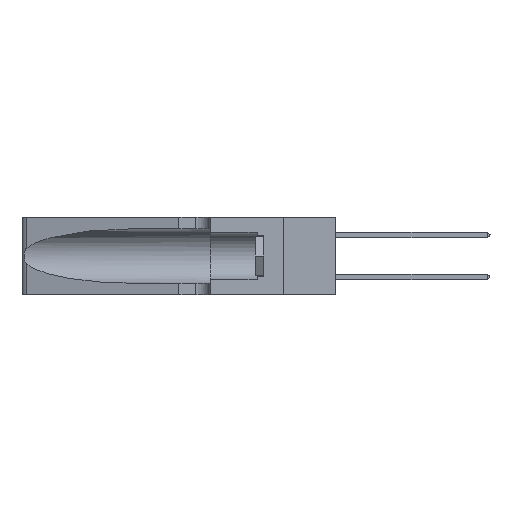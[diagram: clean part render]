
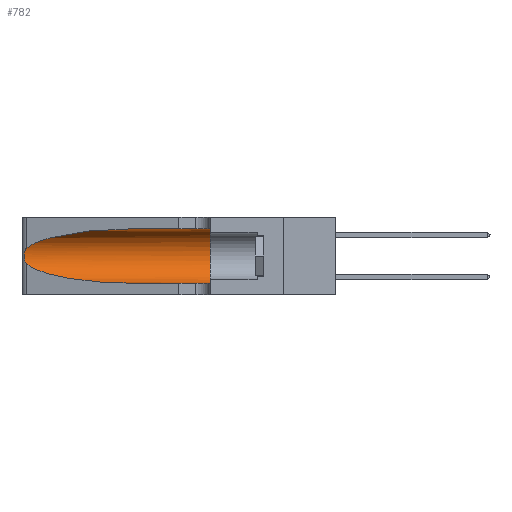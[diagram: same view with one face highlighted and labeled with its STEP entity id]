
A CAD part, left-side view. The second image highlights one B-rep face of the part: STEP entity #782.
In plain terms, the highlighted cylindrical face has radius 3.308 mm (diameter 6.617 mm), a partial arc.
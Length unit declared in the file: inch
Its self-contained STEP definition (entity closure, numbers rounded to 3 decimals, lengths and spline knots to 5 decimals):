
#251 =( BOUNDED_CURVE ( )  B_SPLINE_CURVE ( 3, ( #7441, #18581, #9329, #22350 ),
 .UNSPECIFIED., .F., .F. ) 
 B_SPLINE_CURVE_WITH_KNOTS ( ( 4, 4 ),
 ( 3.44316, 4.71239 ),
 .UNSPECIFIED. ) 
 CURVE ( )  GEOMETRIC_REPRESENTATION_ITEM ( )  RATIONAL_B_SPLINE_CURVE ( ( 1., 0.87, 0.87, 1. ) ) 
 REPRESENTATION_ITEM ( '' )  );
#782 = ADVANCED_FACE ( 'NONE', ( #13911 ), #3469, .F. ) ;
#1122 = VERTEX_POINT ( 'NONE', #4785 ) ;
#1223 = LINE ( 'NONE', #7071, #16036 ) ;
#1306 = ORIENTED_EDGE ( 'NONE', *, *, #3313, .T. ) ;
#1333 = CARTESIAN_POINT ( 'NONE',  ( 0.26075, 1.23896, 0.178 ) ) ;
#2041 =( BOUNDED_CURVE ( )  B_SPLINE_CURVE ( 3, ( #22969, #21087, #9941, #11788 ),
 .UNSPECIFIED., .F., .T. ) 
 B_SPLINE_CURVE_WITH_KNOTS ( ( 4, 4 ),
 ( 1.5708, 2.84003 ),
 .UNSPECIFIED. ) 
 CURVE ( )  GEOMETRIC_REPRESENTATION_ITEM ( )  RATIONAL_B_SPLINE_CURVE ( ( 1., 0.87, 0.87, 1. ) ) 
 REPRESENTATION_ITEM ( '' )  );
#2671 = CIRCLE ( 'NONE', #22895, 0.13025 ) ;
#3184 = CARTESIAN_POINT ( 'NONE',  ( 0.25856, 1.23593, 0.16098 ) ) ;
#3313 = EDGE_CURVE ( 'NONE', #11751, #10967, #2041, .T. ) ;
#3469 = CYLINDRICAL_SURFACE ( 'NONE', #12632, 0.13025 ) ;
#3550 = VERTEX_POINT ( 'NONE', #5030 ) ;
#3907 = ORIENTED_EDGE ( 'NONE', *, *, #18210, .F. ) ;
#4198 = DIRECTION ( 'NONE',  ( 0., -1., 0. ) ) ;
#4785 = CARTESIAN_POINT ( 'NONE',  ( 0.1305, 0.35, 0.31525 ) ) ;
#5030 = CARTESIAN_POINT ( 'NONE',  ( 0.1305, 0.35, 0.05475 ) ) ;
#5050 = CARTESIAN_POINT ( 'NONE',  ( 0.25639, 1.23186, 0.15144 ) ) ;
#5107 = CARTESIAN_POINT ( 'NONE',  ( 0.1305, 0.72297, 0.31525 ) ) ;
#5224 = VERTEX_POINT ( 'NONE', #15531 ) ;
#5407 = EDGE_CURVE ( 'NONE', #10967, #16902, #21883, .T. ) ;
#6035 = DIRECTION ( 'NONE',  ( 0., 1., 0. ) ) ;
#6911 = CARTESIAN_POINT ( 'NONE',  ( 0.25487, 1.22718, 0.14631 ) ) ;
#7071 = CARTESIAN_POINT ( 'NONE',  ( 0.1305, 1.61858, 0.31525 ) ) ;
#7441 = CARTESIAN_POINT ( 'NONE',  ( 0.25487, 1.22718, 0.14631 ) ) ;
#8221 = CARTESIAN_POINT ( 'NONE',  ( 0.25487, 1.22718, 0.22369 ) ) ;
#8714 = CARTESIAN_POINT ( 'NONE',  ( 0.25639, 1.23184, 0.21858 ) ) ;
#9329 = CARTESIAN_POINT ( 'NONE',  ( 0.18966, 0.96281, 0.05475 ) ) ;
#9941 = CARTESIAN_POINT ( 'NONE',  ( 0.2373, 1.15595, 0.28018 ) ) ;
#10300 = ORIENTED_EDGE ( 'NONE', *, *, #14866, .T. ) ;
#10587 = CARTESIAN_POINT ( 'NONE',  ( 0.25854, 1.2359, 0.20912 ) ) ;
#10967 = VERTEX_POINT ( 'NONE', #8221 ) ;
#11233 = CARTESIAN_POINT ( 'NONE',  ( 0.1305, 1.61858, 0.185 ) ) ;
#11715 = LINE ( 'NONE', #19092, #16652 ) ;
#11751 = VERTEX_POINT ( 'NONE', #5107 ) ;
#11788 = CARTESIAN_POINT ( 'NONE',  ( 0.25487, 1.22718, 0.22369 ) ) ;
#12016 = EDGE_LOOP ( 'NONE', ( #1306, #14977, #10300, #21398, #18560, #3907 ) ) ;
#12125 = EDGE_CURVE ( 'NONE', #5224, #3550, #11715, .T. ) ;
#12426 = CARTESIAN_POINT ( 'NONE',  ( 0.26075, 1.23896, 0.19203 ) ) ;
#12547 = CARTESIAN_POINT ( 'NONE',  ( 0.25487, 1.22718, 0.14631 ) ) ;
#12632 = AXIS2_PLACEMENT_3D ( 'NONE', #11233, #16814, #22786 ) ;
#12794 = EDGE_CURVE ( 'NONE', #1122, #3550, #2671, .T. ) ;
#13911 = FACE_OUTER_BOUND ( 'NONE', #12016, .T. ) ;
#14318 = CARTESIAN_POINT ( 'NONE',  ( 0.26017, 1.23833, 0.17102 ) ) ;
#14866 = EDGE_CURVE ( 'NONE', #16902, #5224, #251, .T. ) ;
#14977 = ORIENTED_EDGE ( 'NONE', *, *, #5407, .T. ) ;
#15531 = CARTESIAN_POINT ( 'NONE',  ( 0.1305, 0.72297, 0.05475 ) ) ;
#16036 = VECTOR ( 'NONE', #23860, 39.37008 ) ;
#16101 = CARTESIAN_POINT ( 'NONE',  ( 0.25487, 1.22718, 0.22369 ) ) ;
#16190 = CARTESIAN_POINT ( 'NONE',  ( 0.25789, 1.23486, 0.15765 ) ) ;
#16652 = VECTOR ( 'NONE', #4198, 39.37008 ) ;
#16814 = DIRECTION ( 'NONE',  ( 0., -1., 0. ) ) ;
#16902 = VERTEX_POINT ( 'NONE', #12547 ) ;
#17162 = CARTESIAN_POINT ( 'NONE',  ( 0.1305, 0.35, 0.185 ) ) ;
#18058 = CARTESIAN_POINT ( 'NONE',  ( 0.25555, 1.22993, 0.14849 ) ) ;
#18210 = EDGE_CURVE ( 'NONE', #11751, #1122, #1223, .T. ) ;
#18560 = ORIENTED_EDGE ( 'NONE', *, *, #12794, .F. ) ;
#18581 = CARTESIAN_POINT ( 'NONE',  ( 0.2373, 1.15595, 0.08982 ) ) ;
#19062 = DIRECTION ( 'NONE',  ( 0., 0., 1. ) ) ;
#19092 = CARTESIAN_POINT ( 'NONE',  ( 0.1305, 1.61858, 0.05475 ) ) ;
#19865 = CARTESIAN_POINT ( 'NONE',  ( 0.25555, 1.22994, 0.2215 ) ) ;
#21087 = CARTESIAN_POINT ( 'NONE',  ( 0.18966, 0.96281, 0.31525 ) ) ;
#21398 = ORIENTED_EDGE ( 'NONE', *, *, #12125, .T. ) ;
#21758 = CARTESIAN_POINT ( 'NONE',  ( 0.25787, 1.23484, 0.2124 ) ) ;
#21883 = B_SPLINE_CURVE_WITH_KNOTS ( 'NONE', 3,
 ( #16101, #19865, #8714, #21758, #10587, #23629, #12426, #1333, #14318, #3184, #16190, #5050, #18058, #6911 ),
 .UNSPECIFIED., .F., .F.,
 ( 4, 2, 2, 2, 2, 2, 4 ),
 ( 0., 0.00027, 0.00053, 0.00107, 0.0016, 0.00187, 0.00214 ),
 .UNSPECIFIED. ) ;
#22350 = CARTESIAN_POINT ( 'NONE',  ( 0.1305, 0.72297, 0.05475 ) ) ;
#22786 = DIRECTION ( 'NONE',  ( 0., 0., -1. ) ) ;
#22895 = AXIS2_PLACEMENT_3D ( 'NONE', #17162, #6035, #19062 ) ;
#22969 = CARTESIAN_POINT ( 'NONE',  ( 0.1305, 0.72297, 0.31525 ) ) ;
#23629 = CARTESIAN_POINT ( 'NONE',  ( 0.26018, 1.23835, 0.19895 ) ) ;
#23860 = DIRECTION ( 'NONE',  ( 0., -1., 0. ) ) ;
